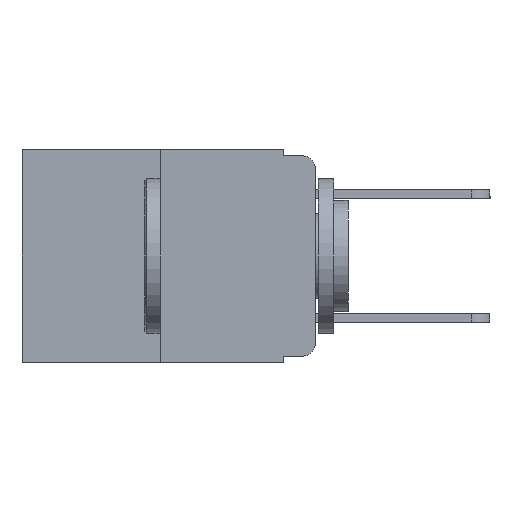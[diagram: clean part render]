
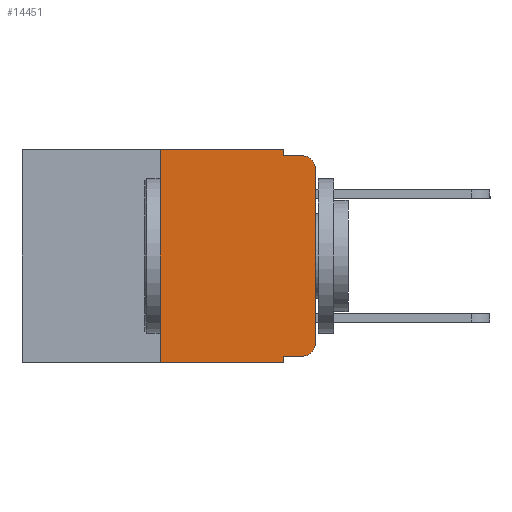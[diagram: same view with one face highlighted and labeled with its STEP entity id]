
A CAD part, left-side view. The second image highlights one B-rep face of the part: STEP entity #14451.
In plain terms, the highlighted planar face has unit normal (-1, 0, 0).
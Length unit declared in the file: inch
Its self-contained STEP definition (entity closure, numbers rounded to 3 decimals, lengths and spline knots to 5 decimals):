
#146 = CIRCLE ( 'NONE', #9552, 0.02 ) ;
#181 = DIRECTION ( 'NONE',  ( 1., 0., 0. ) ) ;
#255 = CARTESIAN_POINT ( 'NONE',  ( 0., 0., 0. ) ) ;
#344 = VERTEX_POINT ( 'NONE', #10056 ) ;
#372 = ORIENTED_EDGE ( 'NONE', *, *, #7803, .T. ) ;
#439 = CARTESIAN_POINT ( 'NONE',  ( 0., 0.473, 0. ) ) ;
#637 = VERTEX_POINT ( 'NONE', #19832 ) ;
#848 = DIRECTION ( 'NONE',  ( 0., 0., -1. ) ) ;
#867 = DIRECTION ( 'NONE',  ( 0., -1., 0. ) ) ;
#1072 = CARTESIAN_POINT ( 'NONE',  ( 0., 0.473, -0.343 ) ) ;
#1137 = CARTESIAN_POINT ( 'NONE',  ( 0., 0.051, 0. ) ) ;
#1331 = CARTESIAN_POINT ( 'NONE',  ( 0., 0.02, -0.03 ) ) ;
#1521 = DIRECTION ( 'NONE',  ( 0., 0., -1. ) ) ;
#1553 = DIRECTION ( 'NONE',  ( -1., 0., 0. ) ) ;
#1906 = EDGE_CURVE ( 'NONE', #4716, #637, #146, .T. ) ;
#2006 = VERTEX_POINT ( 'NONE', #21563 ) ;
#2432 = VECTOR ( 'NONE', #13982, 39.37008 ) ;
#2536 = DIRECTION ( 'NONE',  ( 0., -1., 0. ) ) ;
#2736 = CARTESIAN_POINT ( 'NONE',  ( 0., 0.25, -0.343 ) ) ;
#2857 = LINE ( 'NONE', #439, #18167 ) ;
#3286 = EDGE_CURVE ( 'NONE', #8990, #4716, #13662, .T. ) ;
#3743 = ORIENTED_EDGE ( 'NONE', *, *, #3286, .T. ) ;
#3813 = DIRECTION ( 'NONE',  ( -1., 0., 0. ) ) ;
#4716 = VERTEX_POINT ( 'NONE', #14435 ) ;
#5033 = VERTEX_POINT ( 'NONE', #5479 ) ;
#5307 = LINE ( 'NONE', #1072, #15959 ) ;
#5479 = CARTESIAN_POINT ( 'NONE',  ( 0., 0.02, -0.333 ) ) ;
#5493 = CARTESIAN_POINT ( 'NONE',  ( 0., 0.051, -0.333 ) ) ;
#6168 = DIRECTION ( 'NONE',  ( 0., 0., 1. ) ) ;
#6268 = VECTOR ( 'NONE', #9243, 39.37008 ) ;
#6839 = LINE ( 'NONE', #23425, #12211 ) ;
#7057 = CARTESIAN_POINT ( 'NONE',  ( 0., 0., -0.313 ) ) ;
#7136 = LINE ( 'NONE', #12007, #2432 ) ;
#7803 = EDGE_CURVE ( 'NONE', #5033, #8990, #20727, .T. ) ;
#7995 = CARTESIAN_POINT ( 'NONE',  ( 0., 0.25, 0. ) ) ;
#8562 = ORIENTED_EDGE ( 'NONE', *, *, #21139, .F. ) ;
#8990 = VERTEX_POINT ( 'NONE', #7057 ) ;
#9243 = DIRECTION ( 'NONE',  ( 0., 0., -1. ) ) ;
#9552 = AXIS2_PLACEMENT_3D ( 'NONE', #1331, #1553, #1521 ) ;
#10056 = CARTESIAN_POINT ( 'NONE',  ( 0., 0.051, -0.01 ) ) ;
#11864 = EDGE_CURVE ( 'NONE', #17086, #5033, #12490, .T. ) ;
#11865 = VECTOR ( 'NONE', #867, 39.37008 ) ;
#12007 = CARTESIAN_POINT ( 'NONE',  ( 0., 0.25, 0. ) ) ;
#12211 = VECTOR ( 'NONE', #15561, 39.37008 ) ;
#12296 = CARTESIAN_POINT ( 'NONE',  ( 0., 0.473, 0. ) ) ;
#12490 = LINE ( 'NONE', #20793, #11865 ) ;
#13013 = AXIS2_PLACEMENT_3D ( 'NONE', #12296, #181, #14268 ) ;
#13022 = VECTOR ( 'NONE', #6168, 39.37008 ) ;
#13222 = EDGE_CURVE ( 'NONE', #17086, #18398, #13879, .T. ) ;
#13662 = LINE ( 'NONE', #255, #13022 ) ;
#13879 = LINE ( 'NONE', #20781, #23672 ) ;
#13936 = ORIENTED_EDGE ( 'NONE', *, *, #13222, .F. ) ;
#13982 = DIRECTION ( 'NONE',  ( 0., 0., 1. ) ) ;
#14268 = DIRECTION ( 'NONE',  ( 0., 0., -1. ) ) ;
#14435 = CARTESIAN_POINT ( 'NONE',  ( 0., 0., -0.03 ) ) ;
#14451 = ADVANCED_FACE ( 'NONE', ( #20642 ), #18187, .F. ) ;
#14561 = EDGE_CURVE ( 'NONE', #18689, #2006, #2857, .T. ) ;
#15561 = DIRECTION ( 'NONE',  ( 0., -1., 0. ) ) ;
#15812 = CARTESIAN_POINT ( 'NONE',  ( 0., 0.02, -0.313 ) ) ;
#15906 = AXIS2_PLACEMENT_3D ( 'NONE', #15812, #3813, #17790 ) ;
#15959 = VECTOR ( 'NONE', #21078, 39.37008 ) ;
#16948 = LINE ( 'NONE', #1137, #6268 ) ;
#17086 = VERTEX_POINT ( 'NONE', #5493 ) ;
#17214 = EDGE_CURVE ( 'NONE', #23035, #18689, #7136, .T. ) ;
#17790 = DIRECTION ( 'NONE',  ( 0., 0., -1. ) ) ;
#17939 = ORIENTED_EDGE ( 'NONE', *, *, #1906, .T. ) ;
#18167 = VECTOR ( 'NONE', #2536, 39.37008 ) ;
#18187 = PLANE ( 'NONE',  #13013 ) ;
#18398 = VERTEX_POINT ( 'NONE', #18632 ) ;
#18632 = CARTESIAN_POINT ( 'NONE',  ( 0., 0.051, -0.343 ) ) ;
#18689 = VERTEX_POINT ( 'NONE', #7995 ) ;
#19832 = CARTESIAN_POINT ( 'NONE',  ( 0., 0.02, -0.01 ) ) ;
#19843 = EDGE_CURVE ( 'NONE', #2006, #344, #16948, .T. ) ;
#20508 = EDGE_LOOP ( 'NONE', ( #3743, #17939, #8562, #24005, #25220, #22527, #23138, #13936, #24930, #372 ) ) ;
#20642 = FACE_OUTER_BOUND ( 'NONE', #20508, .T. ) ;
#20727 = CIRCLE ( 'NONE', #15906, 0.02 ) ;
#20781 = CARTESIAN_POINT ( 'NONE',  ( 0., 0.051, 0. ) ) ;
#20793 = CARTESIAN_POINT ( 'NONE',  ( 0., 0.051, -0.333 ) ) ;
#20988 = EDGE_CURVE ( 'NONE', #23035, #18398, #5307, .T. ) ;
#21078 = DIRECTION ( 'NONE',  ( 0., -1., 0. ) ) ;
#21139 = EDGE_CURVE ( 'NONE', #344, #637, #6839, .T. ) ;
#21563 = CARTESIAN_POINT ( 'NONE',  ( 0., 0.051, 0. ) ) ;
#22527 = ORIENTED_EDGE ( 'NONE', *, *, #17214, .F. ) ;
#23035 = VERTEX_POINT ( 'NONE', #2736 ) ;
#23138 = ORIENTED_EDGE ( 'NONE', *, *, #20988, .T. ) ;
#23425 = CARTESIAN_POINT ( 'NONE',  ( 0., 0.051, -0.01 ) ) ;
#23672 = VECTOR ( 'NONE', #848, 39.37008 ) ;
#24005 = ORIENTED_EDGE ( 'NONE', *, *, #19843, .F. ) ;
#24930 = ORIENTED_EDGE ( 'NONE', *, *, #11864, .T. ) ;
#25220 = ORIENTED_EDGE ( 'NONE', *, *, #14561, .F. ) ;
